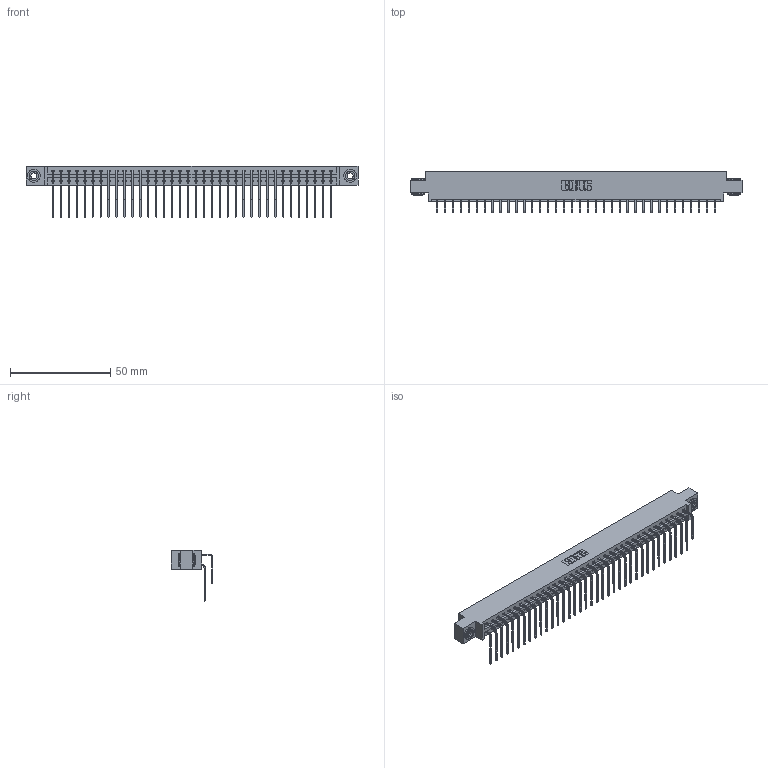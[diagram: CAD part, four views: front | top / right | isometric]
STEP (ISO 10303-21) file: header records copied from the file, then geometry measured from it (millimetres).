
FILE_DESCRIPTION (( 'STEP AP203' ), '1' );
FILE_NAME ('337-072-559-803.STEP', '2018-08-11T15:57:07', ( '' ), ( '' ), 'SwSTEP 2.0', 'SolidWorks 2016', '' );
FILE_SCHEMA (( 'CONFIG_CONTROL_DESIGN' ));
Length unit declared in the file: inch
Products named in the file (5): 337 Part_0.170 Offset - 0.156 Dia-TH; 345-292-001_558 559 Tail - 1; 345-292-001_559 Tail - 2; 345-250-002_345-250-002-102; 337-072-559-803
Assembly tree (75 placements, depth 2):
  337-072-559-803
    337 Part_0.170 Offset - 0.156 Dia-TH
    345-292-001_558 559 Tail - 1  x36
    345-292-001_559 Tail - 2  x36
    345-250-002_345-250-002-102  x2
Bounding box: 165.66 x 20.9 x 25.53 mm (x, y, z)
Volume: 17695.8 mm3; surface area: 22364.7 mm2
Topology: 75 solids, 75 shells, 4188 faces, 12423 edges, 8182 vertices
Faces by surface type: plane 2964, cylinder 1216, cone 8
Entity records: 31254 total; most frequent: CARTESIAN_POINT 5292, ORIENTED_EDGE 5170, DIRECTION 4527, EDGE_CURVE 2585, VECTOR 2393, LINE 2393, VERTEX_POINT 1718, AXIS2_PLACEMENT_3D 1067
